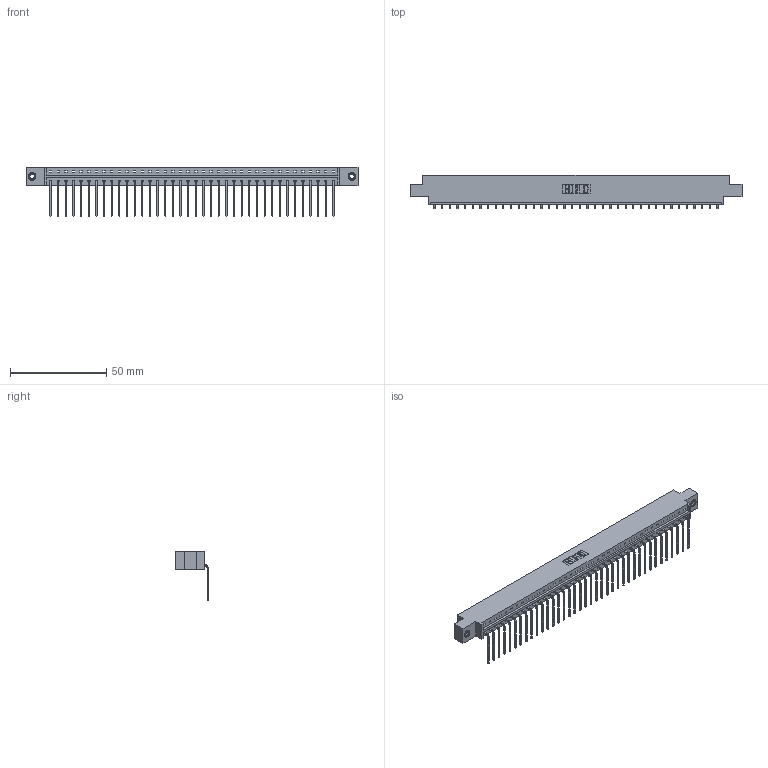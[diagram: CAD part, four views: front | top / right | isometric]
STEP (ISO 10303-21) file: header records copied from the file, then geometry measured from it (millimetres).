
FILE_DESCRIPTION (( 'STEP AP203' ), '1' );
FILE_NAME ('333-038-559-607.STEP', '2018-08-03T12:15:06', ( '' ), ( '' ), 'SwSTEP 2.0', 'SolidWorks 2016', '' );
FILE_SCHEMA (( 'CONFIG_CONTROL_DESIGN' ));
Length unit declared in the file: inch
Products named in the file (4): 333 Part_Offset - .156 Dia - TI; 345-292-001_558 559 Tail - 1; 345-250-001_345-250-005-103; 333-038-559-607
Assembly tree (41 placements, depth 2):
  333-038-559-607
    333 Part_Offset - .156 Dia - TI
    345-292-001_558 559 Tail - 1  x38
    345-250-001_345-250-005-103  x2
Bounding box: 172.11 x 17.09 x 25.53 mm (x, y, z)
Volume: 17170.1 mm3; surface area: 19563.4 mm2
Topology: 41 solids, 41 shells, 2458 faces, 7375 edges, 4858 vertices
Faces by surface type: plane 1778, cylinder 664, cone 12, torus 4
Entity records: 25150 total; most frequent: CARTESIAN_POINT 4323, ORIENTED_EDGE 4290, DIRECTION 3687, EDGE_CURVE 2145, LINE 1997, VECTOR 1997, VERTEX_POINT 1424, AXIS2_PLACEMENT_3D 845
